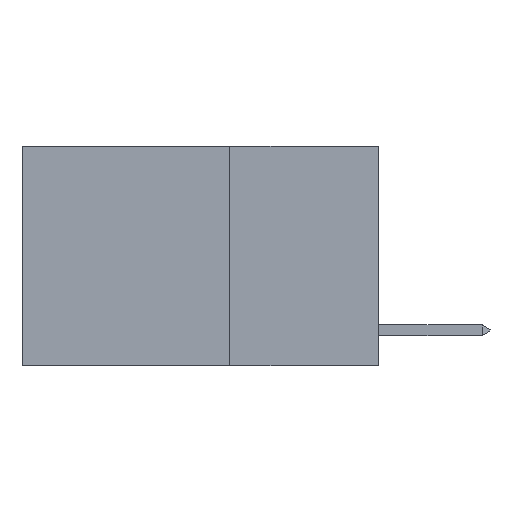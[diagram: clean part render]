
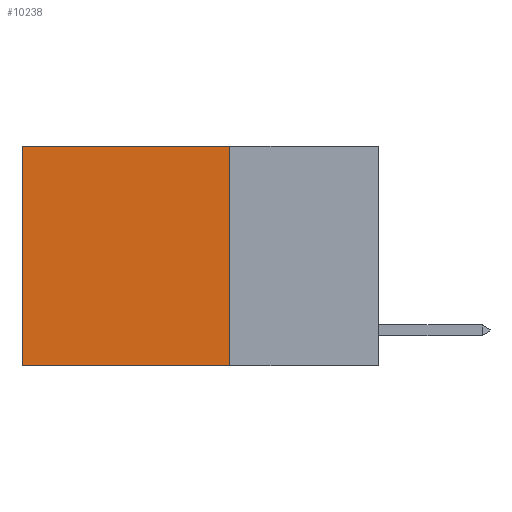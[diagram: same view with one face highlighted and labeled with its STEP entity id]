
A CAD part, left-side view. The second image highlights one B-rep face of the part: STEP entity #10238.
In plain terms, the highlighted planar face has unit normal (-1, 0, 0).
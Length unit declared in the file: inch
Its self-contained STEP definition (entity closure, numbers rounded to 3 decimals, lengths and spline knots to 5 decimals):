
#1591 = DIRECTION ( 'NONE',  ( 0., 1., 0. ) ) ;
#1800 = LINE ( 'NONE', #10103, #25501 ) ;
#2024 = VECTOR ( 'NONE', #1591, 39.37008 ) ;
#2286 = EDGE_LOOP ( 'NONE', ( #20580, #2717, #18255, #11729 ) ) ;
#2717 = ORIENTED_EDGE ( 'NONE', *, *, #16759, .F. ) ;
#3650 = LINE ( 'NONE', #14386, #2024 ) ;
#4906 = LINE ( 'NONE', #11271, #25738 ) ;
#5203 = LINE ( 'NONE', #7389, #8529 ) ;
#6019 = FACE_OUTER_BOUND ( 'NONE', #2286, .T. ) ;
#7389 = CARTESIAN_POINT ( 'NONE',  ( 0.2625, 0.25, 0. ) ) ;
#7664 = CARTESIAN_POINT ( 'NONE',  ( 0.2625, 0.25, -0.37 ) ) ;
#8529 = VECTOR ( 'NONE', #10951, 39.37008 ) ;
#9705 = AXIS2_PLACEMENT_3D ( 'NONE', #12797, #22625, #21096 ) ;
#10103 = CARTESIAN_POINT ( 'NONE',  ( 0.2625, 0.25, 0. ) ) ;
#10238 = ADVANCED_FACE ( 'NONE', ( #6019 ), #18795, .F. ) ;
#10912 = CARTESIAN_POINT ( 'NONE',  ( 0.2625, 0.6, 0. ) ) ;
#10951 = DIRECTION ( 'NONE',  ( 0., 1., 0. ) ) ;
#11271 = CARTESIAN_POINT ( 'NONE',  ( 0.2625, 0.6, 0. ) ) ;
#11729 = ORIENTED_EDGE ( 'NONE', *, *, #14507, .T. ) ;
#12797 = CARTESIAN_POINT ( 'NONE',  ( 0.2625, 0.25, 0. ) ) ;
#13108 = VERTEX_POINT ( 'NONE', #10912 ) ;
#13186 = DIRECTION ( 'NONE',  ( 0., 0., -1. ) ) ;
#13606 = VERTEX_POINT ( 'NONE', #19840 ) ;
#14386 = CARTESIAN_POINT ( 'NONE',  ( 0.2625, 0.25, -0.37 ) ) ;
#14507 = EDGE_CURVE ( 'NONE', #23770, #13108, #5203, .T. ) ;
#16523 = EDGE_CURVE ( 'NONE', #23770, #26651, #1800, .T. ) ;
#16759 = EDGE_CURVE ( 'NONE', #26651, #13606, #3650, .T. ) ;
#18255 = ORIENTED_EDGE ( 'NONE', *, *, #16523, .F. ) ;
#18795 = PLANE ( 'NONE',  #9705 ) ;
#19840 = CARTESIAN_POINT ( 'NONE',  ( 0.2625, 0.6, -0.37 ) ) ;
#20580 = ORIENTED_EDGE ( 'NONE', *, *, #22160, .T. ) ;
#21096 = DIRECTION ( 'NONE',  ( 0., 0., -1. ) ) ;
#22160 = EDGE_CURVE ( 'NONE', #13108, #13606, #4906, .T. ) ;
#22625 = DIRECTION ( 'NONE',  ( 1., 0., 0. ) ) ;
#23380 = DIRECTION ( 'NONE',  ( 0., 0., -1. ) ) ;
#23770 = VERTEX_POINT ( 'NONE', #25163 ) ;
#25163 = CARTESIAN_POINT ( 'NONE',  ( 0.2625, 0.25, 0. ) ) ;
#25501 = VECTOR ( 'NONE', #23380, 39.37008 ) ;
#25738 = VECTOR ( 'NONE', #13186, 39.37008 ) ;
#26651 = VERTEX_POINT ( 'NONE', #7664 ) ;
